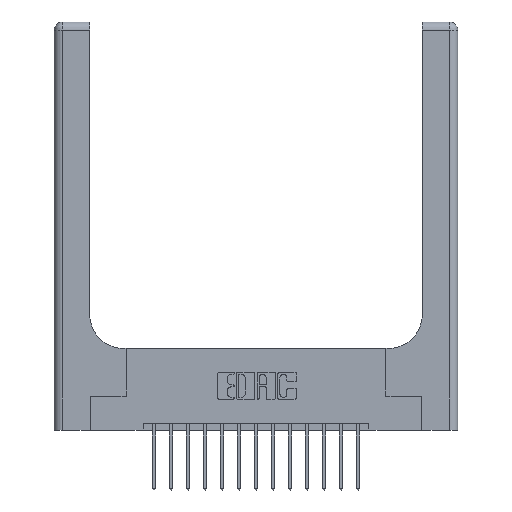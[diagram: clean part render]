
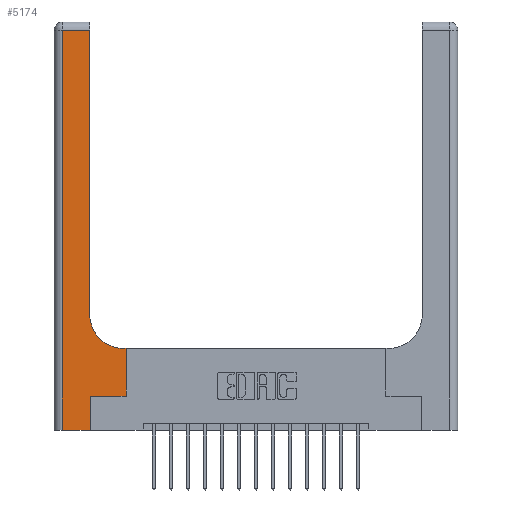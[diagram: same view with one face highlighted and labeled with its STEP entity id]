
A CAD part, top view. The second image highlights one B-rep face of the part: STEP entity #5174.
In plain terms, the highlighted planar face has unit normal (0, 0, 1).
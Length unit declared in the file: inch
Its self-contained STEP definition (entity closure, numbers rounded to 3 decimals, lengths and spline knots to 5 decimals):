
#611 = LINE ( 'NONE', #7922, #9267 ) ;
#1086 = VERTEX_POINT ( 'NONE', #13283 ) ;
#1414 = ORIENTED_EDGE ( 'NONE', *, *, #10504, .T. ) ;
#1525 = ORIENTED_EDGE ( 'NONE', *, *, #3627, .T. ) ;
#2600 = CARTESIAN_POINT ( 'NONE',  ( 0.528, 0.6, 0.37 ) ) ;
#2837 = EDGE_CURVE ( 'NONE', #9957, #11367, #16550, .T. ) ;
#3146 = CARTESIAN_POINT ( 'NONE',  ( 0., 2.94, 0.37 ) ) ;
#3453 = DIRECTION ( 'NONE',  ( 0., 1., 0. ) ) ;
#3524 = DIRECTION ( 'NONE',  ( 0., 0., -1. ) ) ;
#3627 = EDGE_CURVE ( 'NONE', #14267, #7777, #13373, .T. ) ;
#3858 = CARTESIAN_POINT ( 'NONE',  ( 0.26, 0.6, 0.37 ) ) ;
#4040 = CARTESIAN_POINT ( 'NONE',  ( 0.06, 2.94, 0.37 ) ) ;
#4286 = EDGE_CURVE ( 'NONE', #11367, #6695, #7233, .T. ) ;
#4459 = CARTESIAN_POINT ( 'NONE',  ( 0.26, 2.94, 0.37 ) ) ;
#4633 = ORIENTED_EDGE ( 'NONE', *, *, #14877, .T. ) ;
#4757 = DIRECTION ( 'NONE',  ( 0., 1., 0. ) ) ;
#5174 = ADVANCED_FACE ( 'NONE', ( #14611 ), #11985, .F. ) ;
#5380 = EDGE_LOOP ( 'NONE', ( #1525, #17173, #8810, #1414, #4633, #15676, #15996, #13302, #6849 ) ) ;
#5669 = AXIS2_PLACEMENT_3D ( 'NONE', #17499, #14744, #14647 ) ;
#5729 = AXIS2_PLACEMENT_3D ( 'NONE', #13166, #3524, #11808 ) ;
#5797 = LINE ( 'NONE', #11364, #10596 ) ;
#6695 = VERTEX_POINT ( 'NONE', #2600 ) ;
#6704 = VECTOR ( 'NONE', #3453, 39.37008 ) ;
#6849 = ORIENTED_EDGE ( 'NONE', *, *, #18012, .T. ) ;
#7045 = CARTESIAN_POINT ( 'NONE',  ( 0.265, 0., 0.37 ) ) ;
#7233 = LINE ( 'NONE', #12767, #16634 ) ;
#7619 = CARTESIAN_POINT ( 'NONE',  ( 0.26, 0.85, 0.37 ) ) ;
#7777 = VERTEX_POINT ( 'NONE', #4459 ) ;
#7854 = VERTEX_POINT ( 'NONE', #10552 ) ;
#7922 = CARTESIAN_POINT ( 'NONE',  ( 0., 0., 0.37 ) ) ;
#8256 = VERTEX_POINT ( 'NONE', #13173 ) ;
#8419 = EDGE_CURVE ( 'NONE', #7777, #10780, #11359, .T. ) ;
#8810 = ORIENTED_EDGE ( 'NONE', *, *, #15921, .T. ) ;
#9267 = VECTOR ( 'NONE', #13286, 39.37008 ) ;
#9423 = DIRECTION ( 'NONE',  ( -1., 0., 0. ) ) ;
#9957 = VERTEX_POINT ( 'NONE', #17263 ) ;
#10504 = EDGE_CURVE ( 'NONE', #7854, #1086, #611, .T. ) ;
#10552 = CARTESIAN_POINT ( 'NONE',  ( 0.06, 0., 0.37 ) ) ;
#10596 = VECTOR ( 'NONE', #16912, 39.37008 ) ;
#10628 = VECTOR ( 'NONE', #15446, 39.37008 ) ;
#10780 = VERTEX_POINT ( 'NONE', #4040 ) ;
#11359 = LINE ( 'NONE', #3146, #10628 ) ;
#11364 = CARTESIAN_POINT ( 'NONE',  ( 0.06, 3., 0.37 ) ) ;
#11367 = VERTEX_POINT ( 'NONE', #13070 ) ;
#11808 = DIRECTION ( 'NONE',  ( -1., 0., 0. ) ) ;
#11985 = PLANE ( 'NONE',  #5729 ) ;
#12072 = CIRCLE ( 'NONE', #5669, 0.25 ) ;
#12328 = VECTOR ( 'NONE', #15491, 39.37008 ) ;
#12767 = CARTESIAN_POINT ( 'NONE',  ( 0.528, 0.25, 0.37 ) ) ;
#13070 = CARTESIAN_POINT ( 'NONE',  ( 0.528, 0.25, 0.37 ) ) ;
#13166 = CARTESIAN_POINT ( 'NONE',  ( 0., 3., 0.37 ) ) ;
#13173 = CARTESIAN_POINT ( 'NONE',  ( 0.51, 0.6, 0.37 ) ) ;
#13282 = CARTESIAN_POINT ( 'NONE',  ( 0.26, 3., 0.37 ) ) ;
#13283 = CARTESIAN_POINT ( 'NONE',  ( 0.265, 0., 0.37 ) ) ;
#13286 = DIRECTION ( 'NONE',  ( 1., 0., 0. ) ) ;
#13302 = ORIENTED_EDGE ( 'NONE', *, *, #14763, .T. ) ;
#13373 = LINE ( 'NONE', #13282, #6704 ) ;
#14185 = VECTOR ( 'NONE', #15078, 39.37008 ) ;
#14267 = VERTEX_POINT ( 'NONE', #7619 ) ;
#14611 = FACE_OUTER_BOUND ( 'NONE', #5380, .T. ) ;
#14647 = DIRECTION ( 'NONE',  ( 1., 0., 0. ) ) ;
#14744 = DIRECTION ( 'NONE',  ( 0., 0., -1. ) ) ;
#14763 = EDGE_CURVE ( 'NONE', #6695, #8256, #16333, .T. ) ;
#14877 = EDGE_CURVE ( 'NONE', #1086, #9957, #16602, .T. ) ;
#15078 = DIRECTION ( 'NONE',  ( 1., 0., 0. ) ) ;
#15446 = DIRECTION ( 'NONE',  ( -1., 0., 0. ) ) ;
#15491 = DIRECTION ( 'NONE',  ( 0., 1., 0. ) ) ;
#15676 = ORIENTED_EDGE ( 'NONE', *, *, #2837, .T. ) ;
#15921 = EDGE_CURVE ( 'NONE', #10780, #7854, #5797, .T. ) ;
#15996 = ORIENTED_EDGE ( 'NONE', *, *, #4286, .T. ) ;
#16333 = LINE ( 'NONE', #3858, #16696 ) ;
#16550 = LINE ( 'NONE', #17831, #14185 ) ;
#16602 = LINE ( 'NONE', #7045, #12328 ) ;
#16634 = VECTOR ( 'NONE', #4757, 39.37008 ) ;
#16696 = VECTOR ( 'NONE', #9423, 39.37008 ) ;
#16912 = DIRECTION ( 'NONE',  ( 0., -1., 0. ) ) ;
#17173 = ORIENTED_EDGE ( 'NONE', *, *, #8419, .T. ) ;
#17263 = CARTESIAN_POINT ( 'NONE',  ( 0.265, 0.25, 0.37 ) ) ;
#17499 = CARTESIAN_POINT ( 'NONE',  ( 0.51, 0.85, 0.37 ) ) ;
#17831 = CARTESIAN_POINT ( 'NONE',  ( 0.265, 0.25, 0.37 ) ) ;
#18012 = EDGE_CURVE ( 'NONE', #8256, #14267, #12072, .T. ) ;
